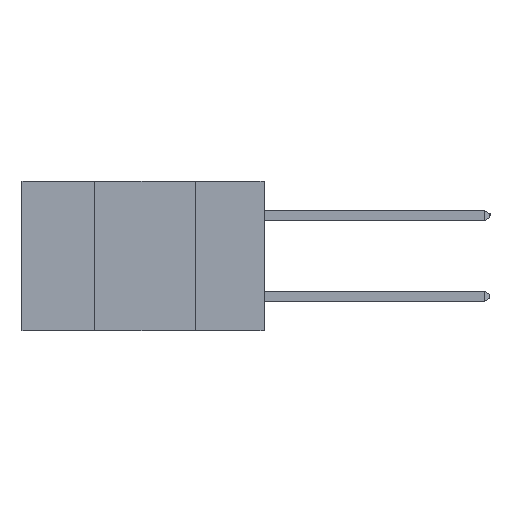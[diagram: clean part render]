
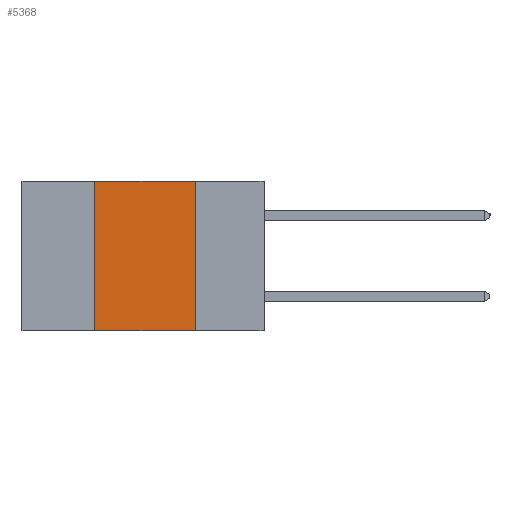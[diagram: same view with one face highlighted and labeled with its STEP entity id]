
A CAD part, left-side view. The second image highlights one B-rep face of the part: STEP entity #5368.
In plain terms, the highlighted planar face has unit normal (-1, 0, 0).
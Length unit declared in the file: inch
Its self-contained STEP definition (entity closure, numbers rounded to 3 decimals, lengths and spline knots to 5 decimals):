
#330 = ORIENTED_EDGE ( 'NONE', *, *, #9090, .F. ) ;
#332 = DIRECTION ( 'NONE',  ( 0., -1., 0. ) ) ;
#361 = DIRECTION ( 'NONE',  ( 0., 0., 1. ) ) ;
#452 = CARTESIAN_POINT ( 'NONE',  ( 0., 0.6, 0. ) ) ;
#1349 = VERTEX_POINT ( 'NONE', #19802 ) ;
#1404 = DIRECTION ( 'NONE',  ( 0., 0., -1. ) ) ;
#2546 = CARTESIAN_POINT ( 'NONE',  ( 0., 0.17, -0.37 ) ) ;
#2864 = DIRECTION ( 'NONE',  ( 0., -1., 0. ) ) ;
#3184 = VERTEX_POINT ( 'NONE', #2546 ) ;
#3678 = PLANE ( 'NONE',  #20266 ) ;
#4036 = ORIENTED_EDGE ( 'NONE', *, *, #8244, .F. ) ;
#5368 = ADVANCED_FACE ( 'NONE', ( #16948 ), #3678, .F. ) ;
#5671 = VECTOR ( 'NONE', #1404, 39.37008 ) ;
#7102 = DIRECTION ( 'NONE',  ( 0., 0., -1. ) ) ;
#7949 = CARTESIAN_POINT ( 'NONE',  ( 0., 0.17, -0.37 ) ) ;
#8244 = EDGE_CURVE ( 'NONE', #17417, #3184, #17685, .T. ) ;
#8498 = LINE ( 'NONE', #15017, #20463 ) ;
#8896 = CARTESIAN_POINT ( 'NONE',  ( 0., 0.42, 0. ) ) ;
#9090 = EDGE_CURVE ( 'NONE', #18584, #17417, #12507, .T. ) ;
#10486 = EDGE_CURVE ( 'NONE', #1349, #3184, #8498, .T. ) ;
#12055 = LINE ( 'NONE', #16859, #13697 ) ;
#12231 = EDGE_LOOP ( 'NONE', ( #4036, #330, #14427, #16778 ) ) ;
#12507 = LINE ( 'NONE', #12722, #17225 ) ;
#12722 = CARTESIAN_POINT ( 'NONE',  ( 0., 0.6, 0. ) ) ;
#13697 = VECTOR ( 'NONE', #361, 39.37008 ) ;
#14427 = ORIENTED_EDGE ( 'NONE', *, *, #14934, .F. ) ;
#14934 = EDGE_CURVE ( 'NONE', #1349, #18584, #12055, .T. ) ;
#15017 = CARTESIAN_POINT ( 'NONE',  ( 0., 0.6, -0.37 ) ) ;
#16778 = ORIENTED_EDGE ( 'NONE', *, *, #10486, .T. ) ;
#16841 = DIRECTION ( 'NONE',  ( 1., 0., 0. ) ) ;
#16859 = CARTESIAN_POINT ( 'NONE',  ( 0., 0.42, -0.37 ) ) ;
#16948 = FACE_OUTER_BOUND ( 'NONE', #12231, .T. ) ;
#17225 = VECTOR ( 'NONE', #2864, 39.37008 ) ;
#17417 = VERTEX_POINT ( 'NONE', #17749 ) ;
#17685 = LINE ( 'NONE', #7949, #5671 ) ;
#17749 = CARTESIAN_POINT ( 'NONE',  ( 0., 0.17, 0. ) ) ;
#18584 = VERTEX_POINT ( 'NONE', #8896 ) ;
#19802 = CARTESIAN_POINT ( 'NONE',  ( 0., 0.42, -0.37 ) ) ;
#20266 = AXIS2_PLACEMENT_3D ( 'NONE', #452, #16841, #7102 ) ;
#20463 = VECTOR ( 'NONE', #332, 39.37008 ) ;
